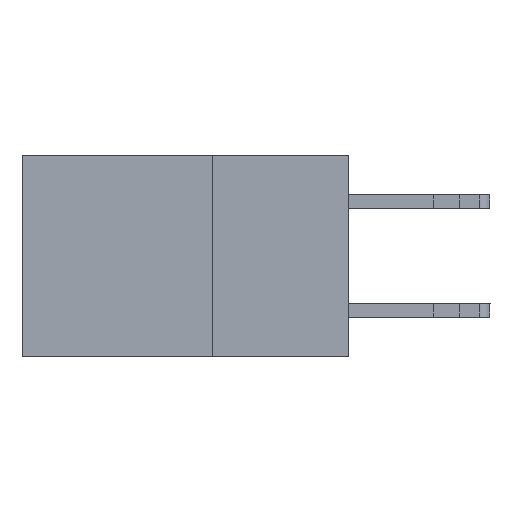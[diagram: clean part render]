
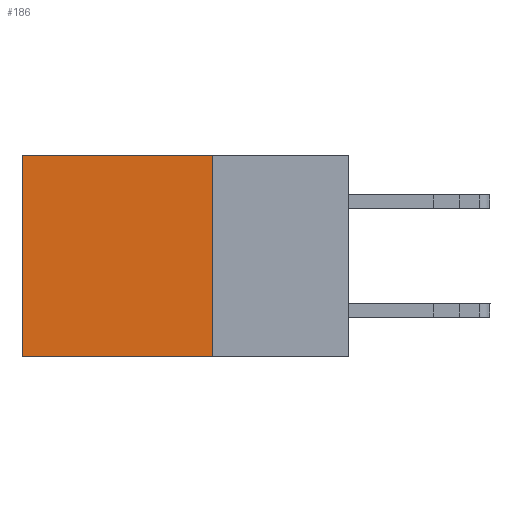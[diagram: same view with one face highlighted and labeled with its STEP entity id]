
A CAD part, left-side view. The second image highlights one B-rep face of the part: STEP entity #186.
In plain terms, the highlighted planar face has unit normal (-1, 0, 0).
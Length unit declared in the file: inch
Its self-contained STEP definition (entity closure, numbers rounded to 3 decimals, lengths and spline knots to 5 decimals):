
#16 = DIRECTION ( 'NONE',  ( 1., 0., 0. ) ) ;
#48 = LINE ( 'NONE', #752, #7451 ) ;
#152 = EDGE_LOOP ( 'NONE', ( #8587, #7287, #11365, #7723 ) ) ;
#186 = ADVANCED_FACE ( 'NONE', ( #421 ), #3749, .F. ) ;
#421 = FACE_OUTER_BOUND ( 'NONE', #152, .T. ) ;
#701 = DIRECTION ( 'NONE',  ( 0., 0., -1. ) ) ;
#716 = VECTOR ( 'NONE', #12452, 39.37008 ) ;
#752 = CARTESIAN_POINT ( 'NONE',  ( 0.2615, 0.25, -0.37 ) ) ;
#769 = CARTESIAN_POINT ( 'NONE',  ( 0.2615, 0.6, -0.37 ) ) ;
#3147 = VERTEX_POINT ( 'NONE', #6311 ) ;
#3749 = PLANE ( 'NONE',  #8354 ) ;
#4253 = VECTOR ( 'NONE', #8657, 39.37008 ) ;
#4627 = VERTEX_POINT ( 'NONE', #769 ) ;
#4756 = EDGE_CURVE ( 'NONE', #9989, #4627, #10212, .T. ) ;
#4766 = CARTESIAN_POINT ( 'NONE',  ( 0.2615, 0.25, -0.37 ) ) ;
#4889 = DIRECTION ( 'NONE',  ( 0., 0., -1. ) ) ;
#6311 = CARTESIAN_POINT ( 'NONE',  ( 0.2615, 0.25, 0. ) ) ;
#6549 = EDGE_CURVE ( 'NONE', #3147, #7705, #14146, .T. ) ;
#7287 = ORIENTED_EDGE ( 'NONE', *, *, #4756, .F. ) ;
#7451 = VECTOR ( 'NONE', #701, 39.37008 ) ;
#7571 = EDGE_CURVE ( 'NONE', #3147, #9989, #48, .T. ) ;
#7705 = VERTEX_POINT ( 'NONE', #9531 ) ;
#7723 = ORIENTED_EDGE ( 'NONE', *, *, #6549, .T. ) ;
#8354 = AXIS2_PLACEMENT_3D ( 'NONE', #11111, #16, #4889 ) ;
#8587 = ORIENTED_EDGE ( 'NONE', *, *, #14803, .T. ) ;
#8657 = DIRECTION ( 'NONE',  ( 0., 1., 0. ) ) ;
#8773 = CARTESIAN_POINT ( 'NONE',  ( 0.2615, 0.25, 0. ) ) ;
#9531 = CARTESIAN_POINT ( 'NONE',  ( 0.2615, 0.6, 0. ) ) ;
#9989 = VERTEX_POINT ( 'NONE', #4766 ) ;
#10066 = LINE ( 'NONE', #12487, #12925 ) ;
#10212 = LINE ( 'NONE', #12432, #716 ) ;
#11111 = CARTESIAN_POINT ( 'NONE',  ( 0.2615, 0.25, -0.37 ) ) ;
#11365 = ORIENTED_EDGE ( 'NONE', *, *, #7571, .F. ) ;
#12432 = CARTESIAN_POINT ( 'NONE',  ( 0.2615, 0.25, -0.37 ) ) ;
#12452 = DIRECTION ( 'NONE',  ( 0., 1., 0. ) ) ;
#12487 = CARTESIAN_POINT ( 'NONE',  ( 0.2615, 0.6, -0.37 ) ) ;
#12925 = VECTOR ( 'NONE', #13670, 39.37008 ) ;
#13670 = DIRECTION ( 'NONE',  ( 0., 0., -1. ) ) ;
#14146 = LINE ( 'NONE', #8773, #4253 ) ;
#14803 = EDGE_CURVE ( 'NONE', #7705, #4627, #10066, .T. ) ;
